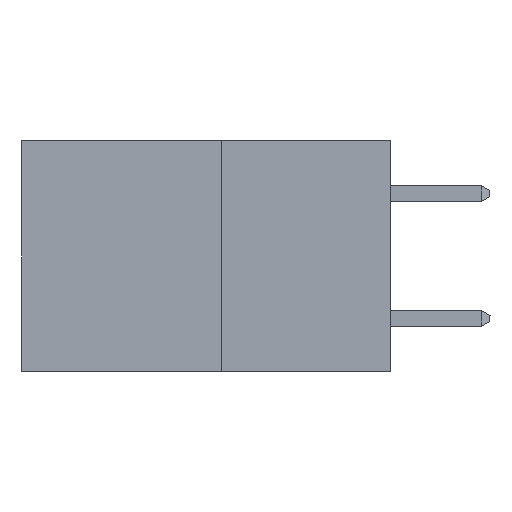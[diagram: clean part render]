
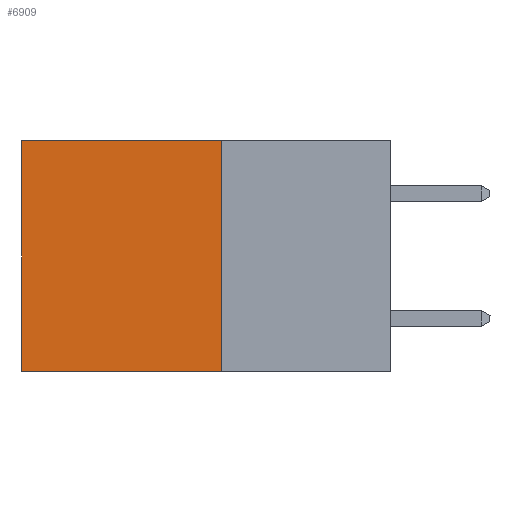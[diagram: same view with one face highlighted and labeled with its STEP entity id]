
A CAD part, left-side view. The second image highlights one B-rep face of the part: STEP entity #6909.
In plain terms, the highlighted planar face has unit normal (-1, 0, 0).
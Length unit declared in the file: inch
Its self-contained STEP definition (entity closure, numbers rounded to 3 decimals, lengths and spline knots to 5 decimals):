
#92 = EDGE_CURVE ( 'NONE', #21922, #13815, #14705, .T. ) ;
#831 = LINE ( 'NONE', #875, #20905 ) ;
#875 = CARTESIAN_POINT ( 'NONE',  ( 0.277, 0.27, 0. ) ) ;
#1394 = DIRECTION ( 'NONE',  ( 1., 0., 0. ) ) ;
#1558 = CARTESIAN_POINT ( 'NONE',  ( 0.277, 0.27, -0.37 ) ) ;
#3089 = VERTEX_POINT ( 'NONE', #13917 ) ;
#4421 = ORIENTED_EDGE ( 'NONE', *, *, #24640, .F. ) ;
#5221 = DIRECTION ( 'NONE',  ( 0., 0., -1. ) ) ;
#6909 = ADVANCED_FACE ( 'NONE', ( #23648 ), #24574, .F. ) ;
#8132 = CARTESIAN_POINT ( 'NONE',  ( 0.277, 0.59, -0.37 ) ) ;
#9603 = VECTOR ( 'NONE', #22493, 39.37008 ) ;
#12439 = VECTOR ( 'NONE', #15235, 39.37008 ) ;
#12613 = DIRECTION ( 'NONE',  ( 0., 1., 0. ) ) ;
#13123 = CARTESIAN_POINT ( 'NONE',  ( 0.277, 0.27, -0.37 ) ) ;
#13319 = ORIENTED_EDGE ( 'NONE', *, *, #21222, .T. ) ;
#13466 = EDGE_LOOP ( 'NONE', ( #13319, #21346, #4421, #17090 ) ) ;
#13815 = VERTEX_POINT ( 'NONE', #8132 ) ;
#13917 = CARTESIAN_POINT ( 'NONE',  ( 0.277, 0.59, 0. ) ) ;
#14705 = LINE ( 'NONE', #16457, #9603 ) ;
#15093 = DIRECTION ( 'NONE',  ( 0., 0., -1. ) ) ;
#15235 = DIRECTION ( 'NONE',  ( 0., 0., -1. ) ) ;
#16005 = LINE ( 'NONE', #16814, #21088 ) ;
#16060 = AXIS2_PLACEMENT_3D ( 'NONE', #13123, #1394, #15093 ) ;
#16457 = CARTESIAN_POINT ( 'NONE',  ( 0.277, 0.27, -0.37 ) ) ;
#16814 = CARTESIAN_POINT ( 'NONE',  ( 0.277, 0.59, -0.37 ) ) ;
#17090 = ORIENTED_EDGE ( 'NONE', *, *, #19162, .T. ) ;
#18910 = VERTEX_POINT ( 'NONE', #21439 ) ;
#19162 = EDGE_CURVE ( 'NONE', #18910, #3089, #831, .T. ) ;
#20574 = CARTESIAN_POINT ( 'NONE',  ( 0.277, 0.27, -0.37 ) ) ;
#20839 = LINE ( 'NONE', #1558, #12439 ) ;
#20905 = VECTOR ( 'NONE', #12613, 39.37008 ) ;
#21088 = VECTOR ( 'NONE', #5221, 39.37008 ) ;
#21222 = EDGE_CURVE ( 'NONE', #3089, #13815, #16005, .T. ) ;
#21346 = ORIENTED_EDGE ( 'NONE', *, *, #92, .F. ) ;
#21439 = CARTESIAN_POINT ( 'NONE',  ( 0.277, 0.27, 0. ) ) ;
#21922 = VERTEX_POINT ( 'NONE', #20574 ) ;
#22493 = DIRECTION ( 'NONE',  ( 0., 1., 0. ) ) ;
#23648 = FACE_OUTER_BOUND ( 'NONE', #13466, .T. ) ;
#24574 = PLANE ( 'NONE',  #16060 ) ;
#24640 = EDGE_CURVE ( 'NONE', #18910, #21922, #20839, .T. ) ;
